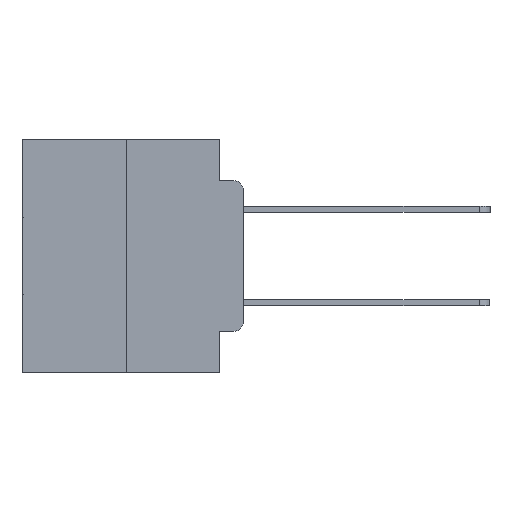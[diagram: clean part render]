
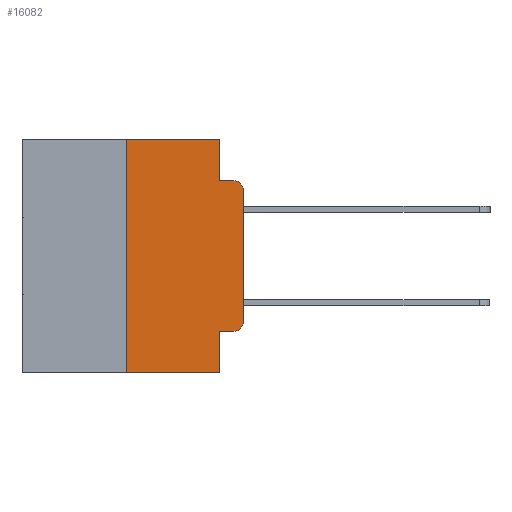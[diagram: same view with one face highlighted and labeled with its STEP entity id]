
A CAD part, left-side view. The second image highlights one B-rep face of the part: STEP entity #16082.
In plain terms, the highlighted planar face has unit normal (-1, 0, 0).
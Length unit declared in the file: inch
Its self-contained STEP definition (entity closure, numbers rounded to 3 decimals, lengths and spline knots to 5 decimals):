
#40 = DIRECTION ( 'NONE',  ( 0., 0., -1. ) ) ;
#1039 = VERTEX_POINT ( 'NONE', #3520 ) ;
#1056 = CARTESIAN_POINT ( 'NONE',  ( 0., 0.051, -0.4115 ) ) ;
#1450 = LINE ( 'NONE', #16456, #18650 ) ;
#2040 = VERTEX_POINT ( 'NONE', #26393 ) ;
#2082 = CARTESIAN_POINT ( 'NONE',  ( 0., 0.02, -0.3915 ) ) ;
#2386 = DIRECTION ( 'NONE',  ( 0., 0., -1. ) ) ;
#2478 = LINE ( 'NONE', #27249, #27178 ) ;
#2639 = FACE_OUTER_BOUND ( 'NONE', #11465, .T. ) ;
#2683 = CARTESIAN_POINT ( 'NONE',  ( 0., 0.051, -0.5 ) ) ;
#3520 = CARTESIAN_POINT ( 'NONE',  ( 0., 0.051, 0. ) ) ;
#3767 = ORIENTED_EDGE ( 'NONE', *, *, #23929, .T. ) ;
#4175 = VERTEX_POINT ( 'NONE', #19849 ) ;
#4527 = DIRECTION ( 'NONE',  ( 0., 0., -1. ) ) ;
#4568 = CARTESIAN_POINT ( 'NONE',  ( 0., 0.02, -0.4115 ) ) ;
#4625 = DIRECTION ( 'NONE',  ( 0., 0., -1. ) ) ;
#5230 = VECTOR ( 'NONE', #13695, 39.37008 ) ;
#5305 = EDGE_CURVE ( 'NONE', #2040, #4175, #2478, .T. ) ;
#6047 = CARTESIAN_POINT ( 'NONE',  ( 0., 0.473, -0.5 ) ) ;
#6117 = LINE ( 'NONE', #24915, #18420 ) ;
#6214 = VERTEX_POINT ( 'NONE', #21725 ) ;
#7517 = ORIENTED_EDGE ( 'NONE', *, *, #17887, .F. ) ;
#9414 = CARTESIAN_POINT ( 'NONE',  ( 0., 0.051, 0. ) ) ;
#9471 = VERTEX_POINT ( 'NONE', #2683 ) ;
#9857 = VECTOR ( 'NONE', #22187, 39.37008 ) ;
#10154 = LINE ( 'NONE', #6047, #21621 ) ;
#11465 = EDGE_LOOP ( 'NONE', ( #26235, #3767, #11599, #29831, #7517, #28031, #23429, #12679, #13404, #14803 ) ) ;
#11559 = CARTESIAN_POINT ( 'NONE',  ( 0., 0., -0.1085 ) ) ;
#11599 = ORIENTED_EDGE ( 'NONE', *, *, #17759, .F. ) ;
#11777 = VERTEX_POINT ( 'NONE', #11559 ) ;
#12679 = ORIENTED_EDGE ( 'NONE', *, *, #24486, .F. ) ;
#12809 = VECTOR ( 'NONE', #27232, 39.37008 ) ;
#13223 = CARTESIAN_POINT ( 'NONE',  ( 0., 0.051, 0. ) ) ;
#13404 = ORIENTED_EDGE ( 'NONE', *, *, #15276, .T. ) ;
#13525 = DIRECTION ( 'NONE',  ( 0., -1., 0. ) ) ;
#13534 = LINE ( 'NONE', #24948, #12809 ) ;
#13606 = CARTESIAN_POINT ( 'NONE',  ( 0., 0.02, -0.0885 ) ) ;
#13695 = DIRECTION ( 'NONE',  ( 0., -1., 0. ) ) ;
#14166 = EDGE_CURVE ( 'NONE', #16920, #11777, #13534, .T. ) ;
#14212 = DIRECTION ( 'NONE',  ( -1., 0., 0. ) ) ;
#14710 = EDGE_CURVE ( 'NONE', #1039, #6214, #15970, .T. ) ;
#14803 = ORIENTED_EDGE ( 'NONE', *, *, #28105, .T. ) ;
#15276 = EDGE_CURVE ( 'NONE', #27821, #25697, #6117, .T. ) ;
#15540 = AXIS2_PLACEMENT_3D ( 'NONE', #20949, #16449, #2386 ) ;
#15785 = LINE ( 'NONE', #9414, #21859 ) ;
#15970 = LINE ( 'NONE', #13223, #9857 ) ;
#16082 = ADVANCED_FACE ( 'NONE', ( #2639 ), #16349, .F. ) ;
#16349 = PLANE ( 'NONE',  #15540 ) ;
#16449 = DIRECTION ( 'NONE',  ( 1., 0., 0. ) ) ;
#16456 = CARTESIAN_POINT ( 'NONE',  ( 0., 0.473, 0. ) ) ;
#16920 = VERTEX_POINT ( 'NONE', #26113 ) ;
#17759 = EDGE_CURVE ( 'NONE', #6214, #22433, #29787, .T. ) ;
#17887 = EDGE_CURVE ( 'NONE', #4175, #1039, #1450, .T. ) ;
#18420 = VECTOR ( 'NONE', #13525, 39.37008 ) ;
#18441 = DIRECTION ( 'NONE',  ( -1., 0., 0. ) ) ;
#18650 = VECTOR ( 'NONE', #23393, 39.37008 ) ;
#19849 = CARTESIAN_POINT ( 'NONE',  ( 0., 0.25, 0. ) ) ;
#19866 = CIRCLE ( 'NONE', #20021, 0.02 ) ;
#19977 = DIRECTION ( 'NONE',  ( 0., -1., 0. ) ) ;
#20021 = AXIS2_PLACEMENT_3D ( 'NONE', #2082, #18441, #4527 ) ;
#20949 = CARTESIAN_POINT ( 'NONE',  ( 0., 0.473, 0. ) ) ;
#21621 = VECTOR ( 'NONE', #19977, 39.37008 ) ;
#21725 = CARTESIAN_POINT ( 'NONE',  ( 0., 0.051, -0.0885 ) ) ;
#21859 = VECTOR ( 'NONE', #4625, 39.37008 ) ;
#22187 = DIRECTION ( 'NONE',  ( 0., 0., -1. ) ) ;
#22433 = VERTEX_POINT ( 'NONE', #13606 ) ;
#22767 = CARTESIAN_POINT ( 'NONE',  ( 0., 0.051, -0.0885 ) ) ;
#23393 = DIRECTION ( 'NONE',  ( 0., -1., 0. ) ) ;
#23429 = ORIENTED_EDGE ( 'NONE', *, *, #29166, .T. ) ;
#23454 = AXIS2_PLACEMENT_3D ( 'NONE', #27891, #14212, #40 ) ;
#23929 = EDGE_CURVE ( 'NONE', #11777, #22433, #24790, .T. ) ;
#24486 = EDGE_CURVE ( 'NONE', #27821, #9471, #15785, .T. ) ;
#24790 = CIRCLE ( 'NONE', #23454, 0.02 ) ;
#24915 = CARTESIAN_POINT ( 'NONE',  ( 0., 0.051, -0.4115 ) ) ;
#24948 = CARTESIAN_POINT ( 'NONE',  ( 0., 0., 0. ) ) ;
#25697 = VERTEX_POINT ( 'NONE', #4568 ) ;
#26113 = CARTESIAN_POINT ( 'NONE',  ( 0., 0., -0.3915 ) ) ;
#26235 = ORIENTED_EDGE ( 'NONE', *, *, #14166, .T. ) ;
#26393 = CARTESIAN_POINT ( 'NONE',  ( 0., 0.25, -0.5 ) ) ;
#27178 = VECTOR ( 'NONE', #27755, 39.37008 ) ;
#27232 = DIRECTION ( 'NONE',  ( 0., 0., 1. ) ) ;
#27249 = CARTESIAN_POINT ( 'NONE',  ( 0., 0.25, 0. ) ) ;
#27755 = DIRECTION ( 'NONE',  ( 0., 0., 1. ) ) ;
#27821 = VERTEX_POINT ( 'NONE', #1056 ) ;
#27891 = CARTESIAN_POINT ( 'NONE',  ( 0., 0.02, -0.1085 ) ) ;
#28031 = ORIENTED_EDGE ( 'NONE', *, *, #5305, .F. ) ;
#28105 = EDGE_CURVE ( 'NONE', #25697, #16920, #19866, .T. ) ;
#29166 = EDGE_CURVE ( 'NONE', #2040, #9471, #10154, .T. ) ;
#29787 = LINE ( 'NONE', #22767, #5230 ) ;
#29831 = ORIENTED_EDGE ( 'NONE', *, *, #14710, .F. ) ;
